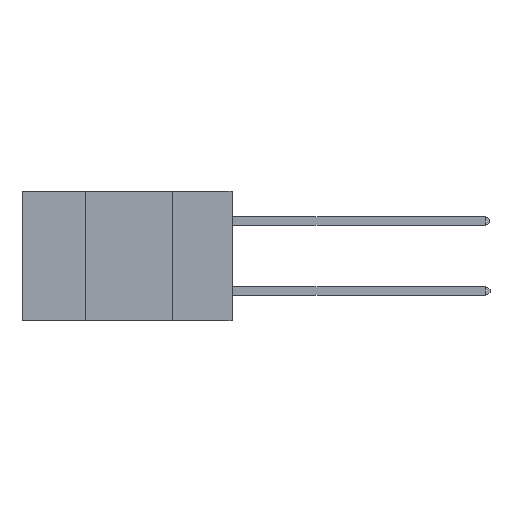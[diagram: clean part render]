
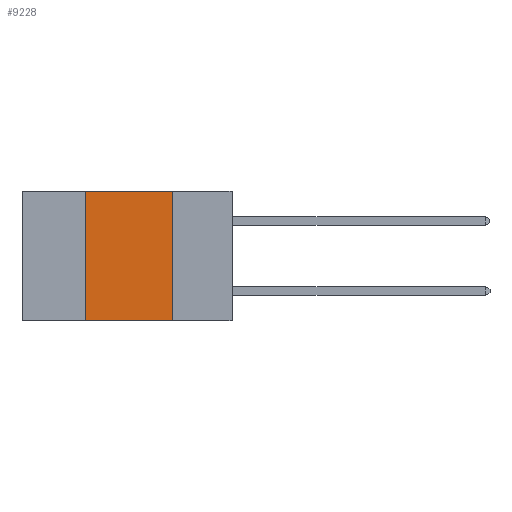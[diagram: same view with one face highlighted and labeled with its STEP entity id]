
A CAD part, left-side view. The second image highlights one B-rep face of the part: STEP entity #9228.
In plain terms, the highlighted planar face has unit normal (-1, 0, 0).
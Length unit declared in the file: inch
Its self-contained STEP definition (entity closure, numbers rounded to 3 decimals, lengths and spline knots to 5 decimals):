
#1009 = DIRECTION ( 'NONE',  ( 0., 0., -1. ) ) ;
#1413 = CARTESIAN_POINT ( 'NONE',  ( 0., 0.17, -0.37 ) ) ;
#1709 = PLANE ( 'NONE',  #9442 ) ;
#2129 = VECTOR ( 'NONE', #1009, 39.37008 ) ;
#2501 = ORIENTED_EDGE ( 'NONE', *, *, #8451, .F. ) ;
#2767 = CARTESIAN_POINT ( 'NONE',  ( 0., 0.42, -0.37 ) ) ;
#4149 = VERTEX_POINT ( 'NONE', #2767 ) ;
#4267 = VERTEX_POINT ( 'NONE', #1413 ) ;
#4355 = EDGE_CURVE ( 'NONE', #16221, #16495, #10622, .T. ) ;
#4990 = EDGE_CURVE ( 'NONE', #4149, #4267, #6118, .T. ) ;
#6118 = LINE ( 'NONE', #17871, #19769 ) ;
#7023 = CARTESIAN_POINT ( 'NONE',  ( 0., 0.42, 0. ) ) ;
#7261 = DIRECTION ( 'NONE',  ( 0., -1., 0. ) ) ;
#7316 = CARTESIAN_POINT ( 'NONE',  ( 0., 0.6, 0. ) ) ;
#8451 = EDGE_CURVE ( 'NONE', #4149, #16221, #13028, .T. ) ;
#8819 = DIRECTION ( 'NONE',  ( 0., 0., 1. ) ) ;
#9228 = ADVANCED_FACE ( 'NONE', ( #20504 ), #1709, .F. ) ;
#9360 = ORIENTED_EDGE ( 'NONE', *, *, #10256, .F. ) ;
#9442 = AXIS2_PLACEMENT_3D ( 'NONE', #7316, #21536, #10870 ) ;
#9742 = CARTESIAN_POINT ( 'NONE',  ( 0., 0.17, 0. ) ) ;
#10256 = EDGE_CURVE ( 'NONE', #16495, #4267, #17658, .T. ) ;
#10622 = LINE ( 'NONE', #19684, #18972 ) ;
#10719 = DIRECTION ( 'NONE',  ( 0., -1., 0. ) ) ;
#10870 = DIRECTION ( 'NONE',  ( 0., 0., -1. ) ) ;
#13028 = LINE ( 'NONE', #7023, #21905 ) ;
#13733 = CARTESIAN_POINT ( 'NONE',  ( 0., 0.17, 0. ) ) ;
#14625 = ORIENTED_EDGE ( 'NONE', *, *, #4990, .T. ) ;
#15466 = EDGE_LOOP ( 'NONE', ( #9360, #17576, #2501, #14625 ) ) ;
#16221 = VERTEX_POINT ( 'NONE', #23137 ) ;
#16495 = VERTEX_POINT ( 'NONE', #9742 ) ;
#17576 = ORIENTED_EDGE ( 'NONE', *, *, #4355, .F. ) ;
#17658 = LINE ( 'NONE', #13733, #2129 ) ;
#17871 = CARTESIAN_POINT ( 'NONE',  ( 0., 0.6, -0.37 ) ) ;
#18972 = VECTOR ( 'NONE', #7261, 39.37008 ) ;
#19684 = CARTESIAN_POINT ( 'NONE',  ( 0., 0.6, 0. ) ) ;
#19769 = VECTOR ( 'NONE', #10719, 39.37008 ) ;
#20504 = FACE_OUTER_BOUND ( 'NONE', #15466, .T. ) ;
#21536 = DIRECTION ( 'NONE',  ( 1., 0., 0. ) ) ;
#21905 = VECTOR ( 'NONE', #8819, 39.37008 ) ;
#23137 = CARTESIAN_POINT ( 'NONE',  ( 0., 0.42, 0. ) ) ;
